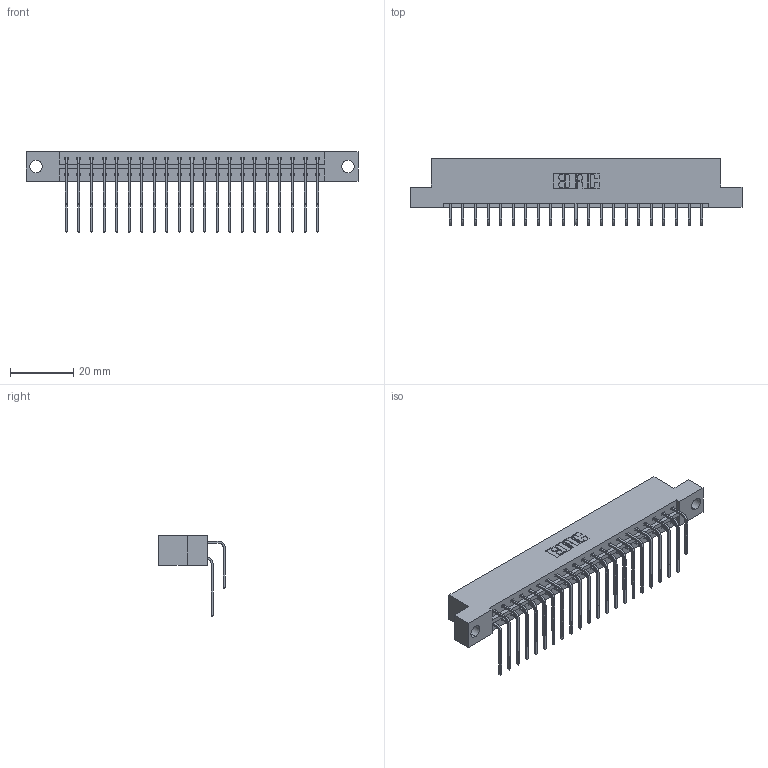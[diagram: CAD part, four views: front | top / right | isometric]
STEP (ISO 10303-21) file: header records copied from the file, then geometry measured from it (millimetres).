
FILE_DESCRIPTION (( 'STEP AP203' ), '1' );
FILE_NAME ('833-042-559-204.STEP', '2020-06-03T22:46:59', ( '' ), ( '' ), 'SwSTEP 2.0', 'SolidWorks 2020', '' );
FILE_SCHEMA (( 'CONFIG_CONTROL_DESIGN' ));
Length unit declared in the file: inch
Products named in the file (4): 345-292-001_559 Tail - 2; 345-292-001_558 559 Tail - 1; 833-042-559-204; 833 Part_Flush - .156 Dia - TH
Assembly tree (43 placements, depth 2):
  833-042-559-204
    833 Part_Flush - .156 Dia - TH
    345-292-001_558 559 Tail - 1  x21
    345-292-001_559 Tail - 2  x21
Bounding box: 104.75 x 20.9 x 25.53 mm (x, y, z)
Volume: 10652.4 mm3; surface area: 13374.4 mm2
Topology: 43 solids, 43 shells, 2382 faces, 7073 edges, 4658 vertices
Faces by surface type: plane 1666, cylinder 716
Entity records: 18013 total; most frequent: CARTESIAN_POINT 3061, ORIENTED_EDGE 2946, DIRECTION 2633, EDGE_CURVE 1473, LINE 1305, VECTOR 1305, VERTEX_POINT 978, AXIS2_PLACEMENT_3D 664
